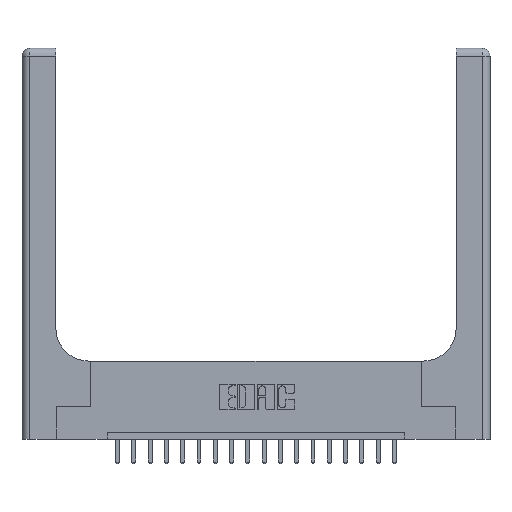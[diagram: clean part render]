
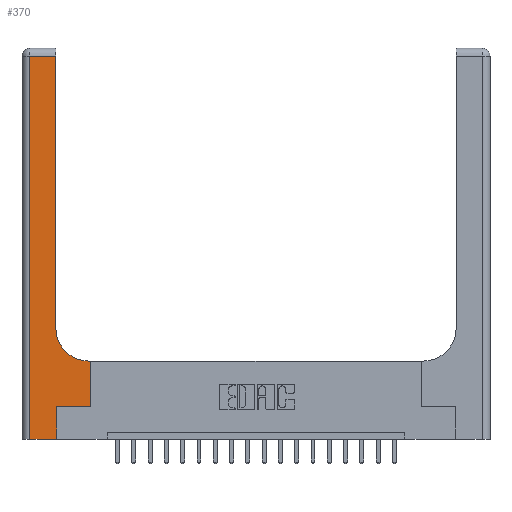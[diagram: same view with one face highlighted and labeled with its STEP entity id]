
A CAD part, top view. The second image highlights one B-rep face of the part: STEP entity #370.
In plain terms, the highlighted planar face has unit normal (0, 0, 1).
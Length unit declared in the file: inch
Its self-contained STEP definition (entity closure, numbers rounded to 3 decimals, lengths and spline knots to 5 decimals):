
#370 = ADVANCED_FACE ( 'NONE', ( #4127 ), #18270, .F. ) ;
#378 = VECTOR ( 'NONE', #14207, 39.37008 ) ;
#959 = DIRECTION ( 'NONE',  ( 0., 1., 0. ) ) ;
#1100 = CARTESIAN_POINT ( 'NONE',  ( 0.06, 3., 0.37 ) ) ;
#1528 = CARTESIAN_POINT ( 'NONE',  ( 0.26, 2.94, 0.37 ) ) ;
#1822 = LINE ( 'NONE', #14257, #12921 ) ;
#1847 = VECTOR ( 'NONE', #18182, 39.37008 ) ;
#1980 = EDGE_LOOP ( 'NONE', ( #11398, #13772, #17377, #16701, #8504, #11561, #3499, #11828, #7116 ) ) ;
#2256 = DIRECTION ( 'NONE',  ( 1., 0., 0. ) ) ;
#2659 = AXIS2_PLACEMENT_3D ( 'NONE', #19520, #11772, #17989 ) ;
#2708 = EDGE_CURVE ( 'NONE', #11260, #19366, #1822, .T. ) ;
#2949 = VERTEX_POINT ( 'NONE', #5992 ) ;
#2978 = LINE ( 'NONE', #15529, #12228 ) ;
#3499 = ORIENTED_EDGE ( 'NONE', *, *, #14528, .T. ) ;
#3943 = VECTOR ( 'NONE', #5586, 39.37008 ) ;
#4127 = FACE_OUTER_BOUND ( 'NONE', #1980, .T. ) ;
#4343 = VERTEX_POINT ( 'NONE', #4963 ) ;
#4501 = CARTESIAN_POINT ( 'NONE',  ( 0.528, 0.25, 0.37 ) ) ;
#4963 = CARTESIAN_POINT ( 'NONE',  ( 0.528, 0.6, 0.37 ) ) ;
#5302 = VECTOR ( 'NONE', #959, 39.37008 ) ;
#5586 = DIRECTION ( 'NONE',  ( 0., -1., 0. ) ) ;
#5677 = VECTOR ( 'NONE', #12122, 39.37008 ) ;
#5945 = DIRECTION ( 'NONE',  ( 0., 0., -1. ) ) ;
#5992 = CARTESIAN_POINT ( 'NONE',  ( 0.265, 0.25, 0.37 ) ) ;
#6656 = CARTESIAN_POINT ( 'NONE',  ( 0.06, 2.94, 0.37 ) ) ;
#7025 = AXIS2_PLACEMENT_3D ( 'NONE', #13682, #5945, #19700 ) ;
#7116 = ORIENTED_EDGE ( 'NONE', *, *, #9317, .T. ) ;
#7831 = CARTESIAN_POINT ( 'NONE',  ( 0.06, 0., 0.37 ) ) ;
#7974 = CARTESIAN_POINT ( 'NONE',  ( 0., 0., 0.37 ) ) ;
#8029 = DIRECTION ( 'NONE',  ( -1., 0., 0. ) ) ;
#8231 = DIRECTION ( 'NONE',  ( 0., 1., 0. ) ) ;
#8504 = ORIENTED_EDGE ( 'NONE', *, *, #12455, .T. ) ;
#8868 = EDGE_CURVE ( 'NONE', #19366, #9766, #10558, .T. ) ;
#9317 = EDGE_CURVE ( 'NONE', #10611, #16234, #9785, .T. ) ;
#9528 = EDGE_CURVE ( 'NONE', #9766, #10136, #15933, .T. ) ;
#9766 = VERTEX_POINT ( 'NONE', #7831 ) ;
#9785 = CIRCLE ( 'NONE', #2659, 0.25 ) ;
#10136 = VERTEX_POINT ( 'NONE', #18825 ) ;
#10558 = LINE ( 'NONE', #1100, #3943 ) ;
#10611 = VERTEX_POINT ( 'NONE', #11233 ) ;
#10702 = EDGE_CURVE ( 'NONE', #16234, #11260, #14925, .T. ) ;
#11233 = CARTESIAN_POINT ( 'NONE',  ( 0.51, 0.6, 0.37 ) ) ;
#11260 = VERTEX_POINT ( 'NONE', #1528 ) ;
#11398 = ORIENTED_EDGE ( 'NONE', *, *, #10702, .T. ) ;
#11561 = ORIENTED_EDGE ( 'NONE', *, *, #19396, .T. ) ;
#11772 = DIRECTION ( 'NONE',  ( 0., 0., -1. ) ) ;
#11828 = ORIENTED_EDGE ( 'NONE', *, *, #16821, .T. ) ;
#12122 = DIRECTION ( 'NONE',  ( 0., 1., 0. ) ) ;
#12228 = VECTOR ( 'NONE', #8231, 39.37008 ) ;
#12455 = EDGE_CURVE ( 'NONE', #10136, #2949, #13658, .T. ) ;
#12921 = VECTOR ( 'NONE', #8029, 39.37008 ) ;
#12966 = VECTOR ( 'NONE', #2256, 39.37008 ) ;
#13159 = CARTESIAN_POINT ( 'NONE',  ( 0.265, 0.25, 0.37 ) ) ;
#13658 = LINE ( 'NONE', #19875, #5677 ) ;
#13682 = CARTESIAN_POINT ( 'NONE',  ( 0., 3., 0.37 ) ) ;
#13772 = ORIENTED_EDGE ( 'NONE', *, *, #2708, .T. ) ;
#14207 = DIRECTION ( 'NONE',  ( 1., 0., 0. ) ) ;
#14257 = CARTESIAN_POINT ( 'NONE',  ( 0., 2.94, 0.37 ) ) ;
#14528 = EDGE_CURVE ( 'NONE', #17318, #4343, #2978, .T. ) ;
#14925 = LINE ( 'NONE', #18364, #5302 ) ;
#15036 = CARTESIAN_POINT ( 'NONE',  ( 0.26, 0.6, 0.37 ) ) ;
#15529 = CARTESIAN_POINT ( 'NONE',  ( 0.528, 0.25, 0.37 ) ) ;
#15933 = LINE ( 'NONE', #7974, #378 ) ;
#16234 = VERTEX_POINT ( 'NONE', #17118 ) ;
#16701 = ORIENTED_EDGE ( 'NONE', *, *, #9528, .T. ) ;
#16821 = EDGE_CURVE ( 'NONE', #4343, #10611, #16845, .T. ) ;
#16845 = LINE ( 'NONE', #15036, #1847 ) ;
#17118 = CARTESIAN_POINT ( 'NONE',  ( 0.26, 0.85, 0.37 ) ) ;
#17318 = VERTEX_POINT ( 'NONE', #4501 ) ;
#17377 = ORIENTED_EDGE ( 'NONE', *, *, #8868, .T. ) ;
#17858 = LINE ( 'NONE', #13159, #12966 ) ;
#17989 = DIRECTION ( 'NONE',  ( 1., 0., 0. ) ) ;
#18182 = DIRECTION ( 'NONE',  ( -1., 0., 0. ) ) ;
#18270 = PLANE ( 'NONE',  #7025 ) ;
#18364 = CARTESIAN_POINT ( 'NONE',  ( 0.26, 3., 0.37 ) ) ;
#18825 = CARTESIAN_POINT ( 'NONE',  ( 0.265, 0., 0.37 ) ) ;
#19366 = VERTEX_POINT ( 'NONE', #6656 ) ;
#19396 = EDGE_CURVE ( 'NONE', #2949, #17318, #17858, .T. ) ;
#19520 = CARTESIAN_POINT ( 'NONE',  ( 0.51, 0.85, 0.37 ) ) ;
#19700 = DIRECTION ( 'NONE',  ( -1., 0., 0. ) ) ;
#19875 = CARTESIAN_POINT ( 'NONE',  ( 0.265, 0., 0.37 ) ) ;
